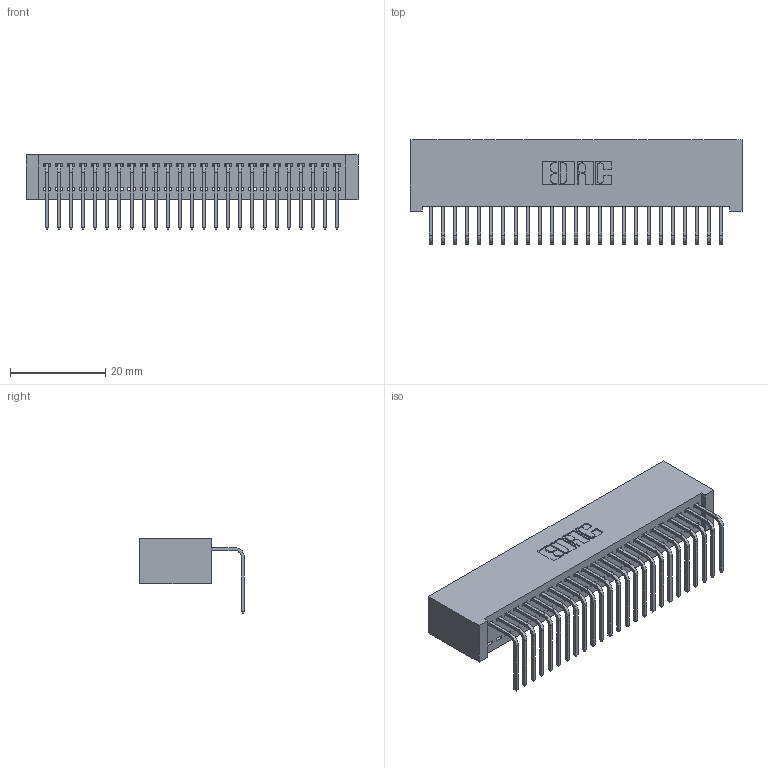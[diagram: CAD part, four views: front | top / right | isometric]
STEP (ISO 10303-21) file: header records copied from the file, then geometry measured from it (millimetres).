
FILE_DESCRIPTION (( 'STEP AP203' ), '1' );
FILE_NAME ('342-025-558-101.STEP', '2019-10-02T00:45:54', ( '' ), ( '' ), 'SwSTEP 2.0', 'SolidWorks 2016', '' );
FILE_SCHEMA (( 'CONFIG_CONTROL_DESIGN' ));
Length unit declared in the file: inch
Products named in the file (3): 342 Part_Lugless; 345-292-001_558 Tail - 2; 342-025-558-101
Assembly tree (26 placements, depth 2):
  342-025-558-101
    342 Part_Lugless
    345-292-001_558 Tail - 2  x25
Bounding box: 69.75 x 21.91 x 15.62 mm (x, y, z)
Volume: 6545.2 mm3; surface area: 10090.2 mm2
Topology: 26 solids, 26 shells, 1602 faces, 4825 edges, 3182 vertices
Faces by surface type: plane 1162, cylinder 440
Entity records: 17157 total; most frequent: CARTESIAN_POINT 2969, ORIENTED_EDGE 2930, DIRECTION 2531, EDGE_CURVE 1465, LINE 1345, VECTOR 1345, VERTEX_POINT 974, AXIS2_PLACEMENT_3D 593
